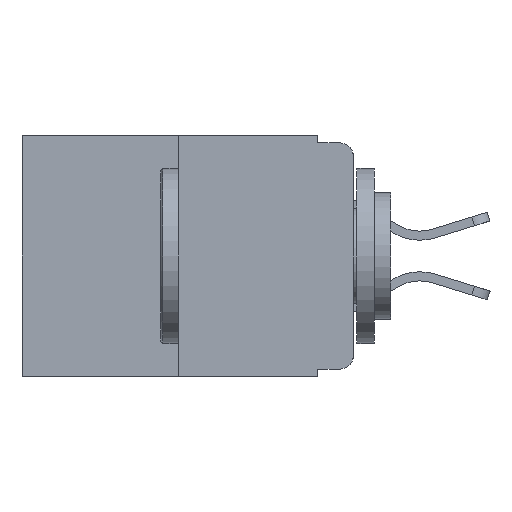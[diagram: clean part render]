
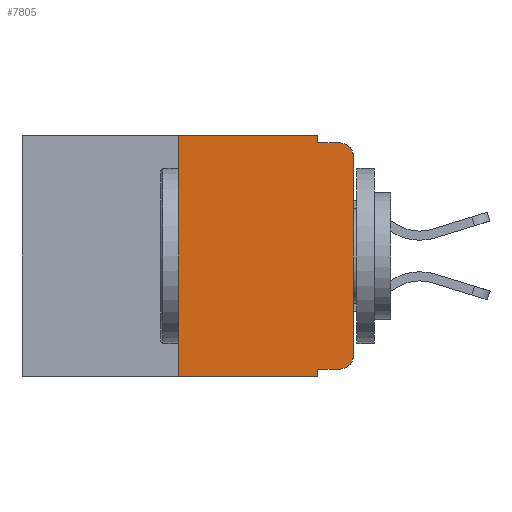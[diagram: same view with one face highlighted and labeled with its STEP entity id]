
A CAD part, left-side view. The second image highlights one B-rep face of the part: STEP entity #7805.
In plain terms, the highlighted planar face has unit normal (-1, 0, 0).
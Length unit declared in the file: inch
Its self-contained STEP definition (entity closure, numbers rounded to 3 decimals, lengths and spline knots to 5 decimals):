
#157 = LINE ( 'NONE', #2818, #14029 ) ;
#183 = CARTESIAN_POINT ( 'NONE',  ( 0., 0.051, 0. ) ) ;
#1219 = CARTESIAN_POINT ( 'NONE',  ( 0., 0.02, -0.313 ) ) ;
#1307 = VERTEX_POINT ( 'NONE', #11227 ) ;
#1476 = EDGE_CURVE ( 'NONE', #6808, #16830, #9008, .T. ) ;
#1501 = VERTEX_POINT ( 'NONE', #6511 ) ;
#1538 = EDGE_CURVE ( 'NONE', #18404, #18203, #9549, .T. ) ;
#1759 = CARTESIAN_POINT ( 'NONE',  ( 0., 0.25, 0. ) ) ;
#2224 = ORIENTED_EDGE ( 'NONE', *, *, #1476, .F. ) ;
#2345 = CARTESIAN_POINT ( 'NONE',  ( 0., 0.051, -0.01 ) ) ;
#2451 = ORIENTED_EDGE ( 'NONE', *, *, #3344, .F. ) ;
#2807 = VECTOR ( 'NONE', #5296, 39.37008 ) ;
#2818 = CARTESIAN_POINT ( 'NONE',  ( 0., 0.25, 0. ) ) ;
#3344 = EDGE_CURVE ( 'NONE', #18227, #1307, #12135, .T. ) ;
#3474 = ORIENTED_EDGE ( 'NONE', *, *, #11500, .T. ) ;
#3897 = ORIENTED_EDGE ( 'NONE', *, *, #5911, .T. ) ;
#4047 = CIRCLE ( 'NONE', #14542, 0.02 ) ;
#4528 = ORIENTED_EDGE ( 'NONE', *, *, #10965, .T. ) ;
#4664 = LINE ( 'NONE', #11687, #6444 ) ;
#4876 = VECTOR ( 'NONE', #5026, 39.37008 ) ;
#5007 = CARTESIAN_POINT ( 'NONE',  ( 0., 0.051, -0.01 ) ) ;
#5026 = DIRECTION ( 'NONE',  ( 0., 0., -1. ) ) ;
#5296 = DIRECTION ( 'NONE',  ( 0., 0., -1. ) ) ;
#5356 = FACE_OUTER_BOUND ( 'NONE', #13961, .T. ) ;
#5911 = EDGE_CURVE ( 'NONE', #16064, #18203, #7823, .T. ) ;
#6409 = ORIENTED_EDGE ( 'NONE', *, *, #15880, .F. ) ;
#6444 = VECTOR ( 'NONE', #7570, 39.37008 ) ;
#6511 = CARTESIAN_POINT ( 'NONE',  ( 0., 0.02, -0.333 ) ) ;
#6599 = CARTESIAN_POINT ( 'NONE',  ( 0., 0.051, 0. ) ) ;
#6808 = VERTEX_POINT ( 'NONE', #1759 ) ;
#7412 = CARTESIAN_POINT ( 'NONE',  ( 0., 0., -0.03 ) ) ;
#7523 = DIRECTION ( 'NONE',  ( -1., 0., 0. ) ) ;
#7570 = DIRECTION ( 'NONE',  ( 0., -1., 0. ) ) ;
#7805 = ADVANCED_FACE ( 'NONE', ( #5356 ), #16639, .F. ) ;
#7813 = CARTESIAN_POINT ( 'NONE',  ( 0., 0.051, -0.343 ) ) ;
#7823 = LINE ( 'NONE', #9077, #7951 ) ;
#7951 = VECTOR ( 'NONE', #9347, 39.37008 ) ;
#8028 = LINE ( 'NONE', #6599, #2807 ) ;
#8098 = VERTEX_POINT ( 'NONE', #7412 ) ;
#8282 = DIRECTION ( 'NONE',  ( 1., 0., 0. ) ) ;
#8472 = ORIENTED_EDGE ( 'NONE', *, *, #11020, .T. ) ;
#8622 = CARTESIAN_POINT ( 'NONE',  ( 0., 0., 0. ) ) ;
#8772 = CARTESIAN_POINT ( 'NONE',  ( 0., 0.02, -0.03 ) ) ;
#9008 = LINE ( 'NONE', #17539, #9693 ) ;
#9077 = CARTESIAN_POINT ( 'NONE',  ( 0., 0.473, -0.343 ) ) ;
#9347 = DIRECTION ( 'NONE',  ( 0., -1., 0. ) ) ;
#9549 = LINE ( 'NONE', #11123, #4876 ) ;
#9611 = DIRECTION ( 'NONE',  ( -1., 0., 0. ) ) ;
#9655 = ORIENTED_EDGE ( 'NONE', *, *, #10293, .F. ) ;
#9693 = VECTOR ( 'NONE', #14704, 39.37008 ) ;
#9932 = AXIS2_PLACEMENT_3D ( 'NONE', #16827, #8282, #13992 ) ;
#10169 = DIRECTION ( 'NONE',  ( 0., 0., -1. ) ) ;
#10228 = CARTESIAN_POINT ( 'NONE',  ( 0., 0.051, -0.333 ) ) ;
#10293 = EDGE_CURVE ( 'NONE', #16830, #18227, #8028, .T. ) ;
#10368 = VECTOR ( 'NONE', #16484, 39.37008 ) ;
#10649 = AXIS2_PLACEMENT_3D ( 'NONE', #8772, #7523, #10169 ) ;
#10811 = VERTEX_POINT ( 'NONE', #14860 ) ;
#10965 = EDGE_CURVE ( 'NONE', #1501, #10811, #4047, .T. ) ;
#11020 = EDGE_CURVE ( 'NONE', #8098, #1307, #16962, .T. ) ;
#11101 = DIRECTION ( 'NONE',  ( 0., 0., -1. ) ) ;
#11123 = CARTESIAN_POINT ( 'NONE',  ( 0., 0.051, 0. ) ) ;
#11227 = CARTESIAN_POINT ( 'NONE',  ( 0., 0.02, -0.01 ) ) ;
#11500 = EDGE_CURVE ( 'NONE', #18404, #1501, #4664, .T. ) ;
#11687 = CARTESIAN_POINT ( 'NONE',  ( 0., 0.051, -0.333 ) ) ;
#11831 = CARTESIAN_POINT ( 'NONE',  ( 0., 0.25, -0.343 ) ) ;
#12135 = LINE ( 'NONE', #5007, #10368 ) ;
#12850 = ORIENTED_EDGE ( 'NONE', *, *, #1538, .F. ) ;
#12888 = VECTOR ( 'NONE', #18292, 39.37008 ) ;
#13961 = EDGE_LOOP ( 'NONE', ( #14595, #8472, #2451, #9655, #2224, #6409, #3897, #12850, #3474, #4528 ) ) ;
#13992 = DIRECTION ( 'NONE',  ( 0., 0., -1. ) ) ;
#14029 = VECTOR ( 'NONE', #17391, 39.37008 ) ;
#14542 = AXIS2_PLACEMENT_3D ( 'NONE', #1219, #9611, #11101 ) ;
#14595 = ORIENTED_EDGE ( 'NONE', *, *, #17476, .T. ) ;
#14704 = DIRECTION ( 'NONE',  ( 0., -1., 0. ) ) ;
#14860 = CARTESIAN_POINT ( 'NONE',  ( 0., 0., -0.313 ) ) ;
#15650 = LINE ( 'NONE', #8622, #12888 ) ;
#15880 = EDGE_CURVE ( 'NONE', #16064, #6808, #157, .T. ) ;
#16064 = VERTEX_POINT ( 'NONE', #11831 ) ;
#16484 = DIRECTION ( 'NONE',  ( 0., -1., 0. ) ) ;
#16639 = PLANE ( 'NONE',  #9932 ) ;
#16827 = CARTESIAN_POINT ( 'NONE',  ( 0., 0.473, 0. ) ) ;
#16830 = VERTEX_POINT ( 'NONE', #183 ) ;
#16962 = CIRCLE ( 'NONE', #10649, 0.02 ) ;
#17391 = DIRECTION ( 'NONE',  ( 0., 0., 1. ) ) ;
#17476 = EDGE_CURVE ( 'NONE', #10811, #8098, #15650, .T. ) ;
#17539 = CARTESIAN_POINT ( 'NONE',  ( 0., 0.473, 0. ) ) ;
#18203 = VERTEX_POINT ( 'NONE', #7813 ) ;
#18227 = VERTEX_POINT ( 'NONE', #2345 ) ;
#18292 = DIRECTION ( 'NONE',  ( 0., 0., 1. ) ) ;
#18404 = VERTEX_POINT ( 'NONE', #10228 ) ;
